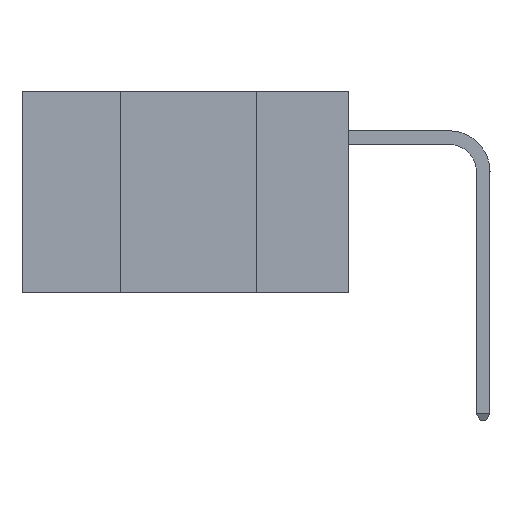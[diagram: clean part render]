
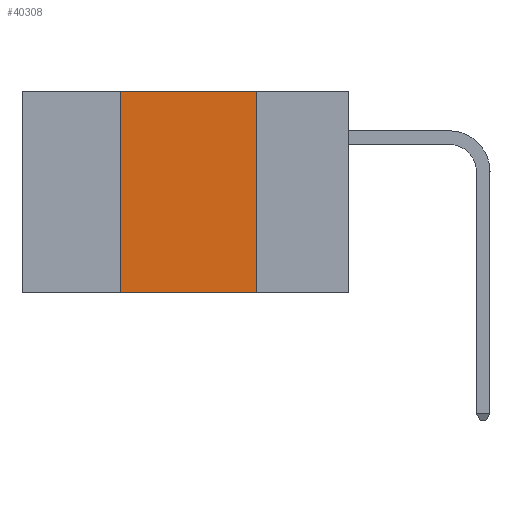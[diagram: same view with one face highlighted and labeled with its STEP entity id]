
A CAD part, left-side view. The second image highlights one B-rep face of the part: STEP entity #40308.
In plain terms, the highlighted planar face has unit normal (-1, 0, 0).
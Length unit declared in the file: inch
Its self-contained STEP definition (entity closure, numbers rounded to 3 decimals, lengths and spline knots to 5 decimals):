
#998 = CARTESIAN_POINT ( 'NONE',  ( 0., 0.6, 0. ) ) ;
#3188 = ORIENTED_EDGE ( 'NONE', *, *, #44057, .T. ) ;
#4490 = DIRECTION ( 'NONE',  ( 0., 0., -1. ) ) ;
#5072 = CARTESIAN_POINT ( 'NONE',  ( 0., 0.42, 0. ) ) ;
#5691 = DIRECTION ( 'NONE',  ( 0., -1., 0. ) ) ;
#6492 = CARTESIAN_POINT ( 'NONE',  ( 0., 0.17, 0. ) ) ;
#6506 = CARTESIAN_POINT ( 'NONE',  ( 0., 0.42, -0.37 ) ) ;
#8591 = DIRECTION ( 'NONE',  ( 0., 0., 1. ) ) ;
#8594 = LINE ( 'NONE', #18428, #18006 ) ;
#10306 = EDGE_CURVE ( 'NONE', #17373, #18192, #42332, .T. ) ;
#14557 = CARTESIAN_POINT ( 'NONE',  ( 0., 0.6, 0. ) ) ;
#15063 = EDGE_CURVE ( 'NONE', #41711, #19604, #8594, .T. ) ;
#16253 = VECTOR ( 'NONE', #35565, 39.37008 ) ;
#16354 = CARTESIAN_POINT ( 'NONE',  ( 0., 0.6, -0.37 ) ) ;
#17373 = VERTEX_POINT ( 'NONE', #6506 ) ;
#18006 = VECTOR ( 'NONE', #35875, 39.37008 ) ;
#18192 = VERTEX_POINT ( 'NONE', #36263 ) ;
#18428 = CARTESIAN_POINT ( 'NONE',  ( 0., 0.17, 0. ) ) ;
#18524 = PLANE ( 'NONE',  #29841 ) ;
#19404 = VECTOR ( 'NONE', #8591, 39.37008 ) ;
#19604 = VERTEX_POINT ( 'NONE', #39950 ) ;
#22469 = ORIENTED_EDGE ( 'NONE', *, *, #15063, .F. ) ;
#22533 = LINE ( 'NONE', #16354, #41101 ) ;
#24079 = FACE_OUTER_BOUND ( 'NONE', #28277, .T. ) ;
#25609 = DIRECTION ( 'NONE',  ( 1., 0., 0. ) ) ;
#28277 = EDGE_LOOP ( 'NONE', ( #22469, #41033, #35038, #3188 ) ) ;
#29841 = AXIS2_PLACEMENT_3D ( 'NONE', #998, #25609, #4490 ) ;
#35038 = ORIENTED_EDGE ( 'NONE', *, *, #10306, .F. ) ;
#35565 = DIRECTION ( 'NONE',  ( 0., -1., 0. ) ) ;
#35875 = DIRECTION ( 'NONE',  ( 0., 0., -1. ) ) ;
#36263 = CARTESIAN_POINT ( 'NONE',  ( 0., 0.42, 0. ) ) ;
#39950 = CARTESIAN_POINT ( 'NONE',  ( 0., 0.17, -0.37 ) ) ;
#40308 = ADVANCED_FACE ( 'NONE', ( #24079 ), #18524, .F. ) ;
#41033 = ORIENTED_EDGE ( 'NONE', *, *, #41279, .F. ) ;
#41101 = VECTOR ( 'NONE', #5691, 39.37008 ) ;
#41279 = EDGE_CURVE ( 'NONE', #18192, #41711, #44132, .T. ) ;
#41711 = VERTEX_POINT ( 'NONE', #6492 ) ;
#42332 = LINE ( 'NONE', #5072, #19404 ) ;
#44057 = EDGE_CURVE ( 'NONE', #17373, #19604, #22533, .T. ) ;
#44132 = LINE ( 'NONE', #14557, #16253 ) ;
